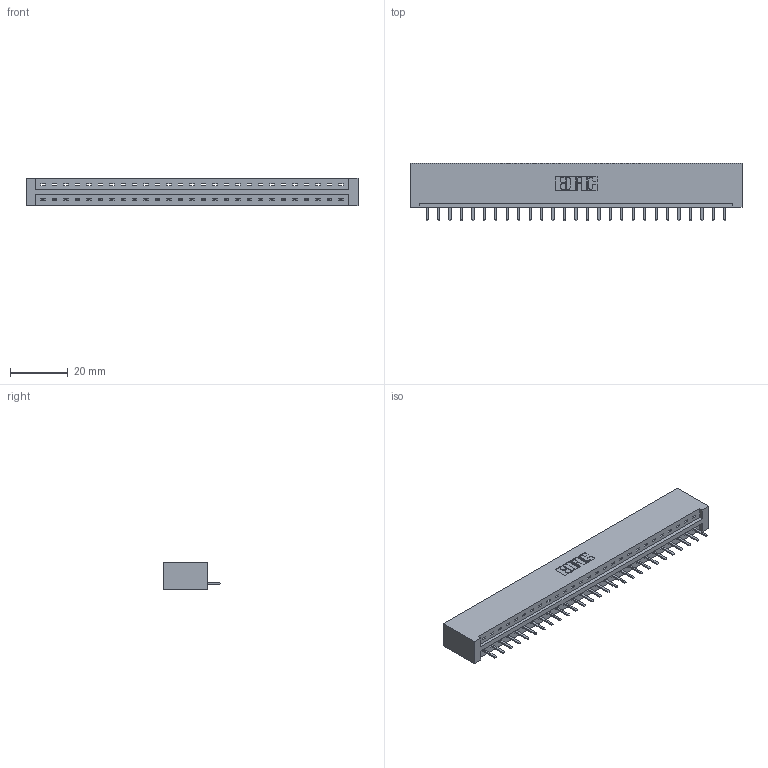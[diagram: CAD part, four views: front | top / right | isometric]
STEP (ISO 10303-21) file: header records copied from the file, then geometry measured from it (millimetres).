
FILE_DESCRIPTION (( 'STEP AP203' ), '1' );
FILE_NAME ('387-027-520-101.STEP', '2018-09-16T13:28:06', ( '' ), ( '' ), 'SwSTEP 2.0', 'SolidWorks 2016', '' );
FILE_SCHEMA (( 'CONFIG_CONTROL_DESIGN' ));
Length unit declared in the file: inch
Products named in the file (3): 337 Part_No Mounting Lugs; 345-292-001_345-293-120; 387-027-520-101
Assembly tree (28 placements, depth 2):
  387-027-520-101
    337 Part_No Mounting Lugs
    345-292-001_345-293-120  x27
Bounding box: 114.86 x 20.02 x 9.4 mm (x, y, z)
Volume: 12411 mm3; surface area: 12443.5 mm2
Topology: 28 solids, 28 shells, 1888 faces, 5579 edges, 3646 vertices
Faces by surface type: plane 1362, cylinder 526
Entity records: 21847 total; most frequent: CARTESIAN_POINT 3823, ORIENTED_EDGE 3774, DIRECTION 3229, EDGE_CURVE 1887, VECTOR 1763, LINE 1763, VERTEX_POINT 1254, AXIS2_PLACEMENT_3D 733
